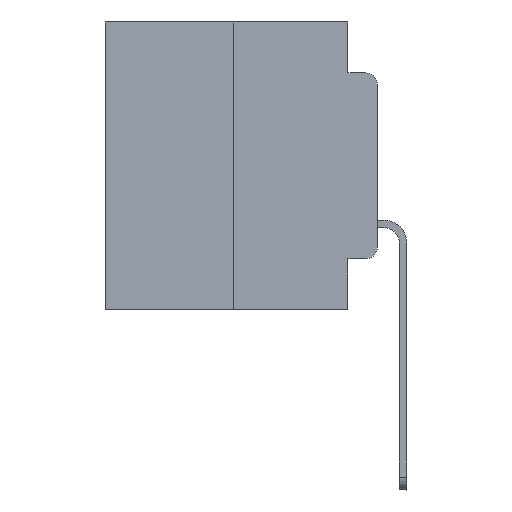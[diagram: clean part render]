
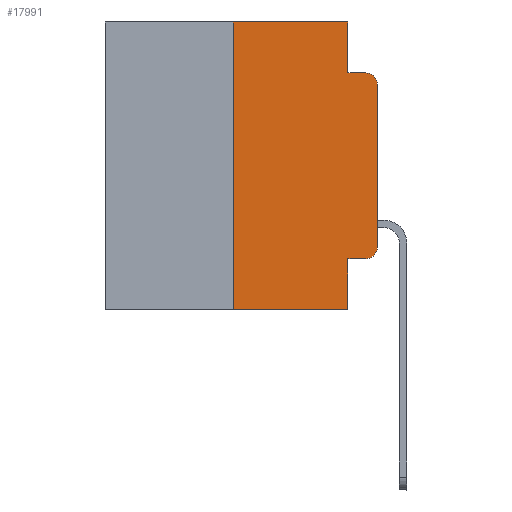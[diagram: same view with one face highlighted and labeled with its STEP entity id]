
A CAD part, left-side view. The second image highlights one B-rep face of the part: STEP entity #17991.
In plain terms, the highlighted planar face has unit normal (-1, 0, 0).
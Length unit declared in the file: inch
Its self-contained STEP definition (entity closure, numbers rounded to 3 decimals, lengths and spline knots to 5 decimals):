
#566 = CARTESIAN_POINT ( 'NONE',  ( 0., 0.051, 0. ) ) ;
#1534 = ORIENTED_EDGE ( 'NONE', *, *, #21400, .T. ) ;
#1569 = LINE ( 'NONE', #5666, #11738 ) ;
#3071 = CARTESIAN_POINT ( 'NONE',  ( 0., 0.02, -0.1085 ) ) ;
#3214 = DIRECTION ( 'NONE',  ( 0., -1., 0. ) ) ;
#3222 = DIRECTION ( 'NONE',  ( 0., 0., -1. ) ) ;
#3319 = VERTEX_POINT ( 'NONE', #20977 ) ;
#3355 = DIRECTION ( 'NONE',  ( -1., 0., 0. ) ) ;
#3459 = EDGE_CURVE ( 'NONE', #23044, #3319, #19981, .T. ) ;
#3983 = EDGE_CURVE ( 'NONE', #18690, #12984, #22580, .T. ) ;
#4078 = ORIENTED_EDGE ( 'NONE', *, *, #25641, .F. ) ;
#4236 = VECTOR ( 'NONE', #19928, 39.37008 ) ;
#4515 = DIRECTION ( 'NONE',  ( 0., 0., -1. ) ) ;
#4939 = CARTESIAN_POINT ( 'NONE',  ( 0., 0.25, 0. ) ) ;
#5666 = CARTESIAN_POINT ( 'NONE',  ( 0., 0.473, -0.5 ) ) ;
#6993 = ORIENTED_EDGE ( 'NONE', *, *, #23756, .F. ) ;
#7085 = CARTESIAN_POINT ( 'NONE',  ( 0., 0.051, -0.5 ) ) ;
#7463 = CARTESIAN_POINT ( 'NONE',  ( 0., 0., -0.3915 ) ) ;
#7580 = CARTESIAN_POINT ( 'NONE',  ( 0., 0.02, -0.4115 ) ) ;
#8139 = DIRECTION ( 'NONE',  ( 0., -1., 0. ) ) ;
#8253 = CARTESIAN_POINT ( 'NONE',  ( 0., 0.051, 0. ) ) ;
#8683 = EDGE_CURVE ( 'NONE', #12984, #23044, #17584, .T. ) ;
#8692 = FACE_OUTER_BOUND ( 'NONE', #15921, .T. ) ;
#8876 = CARTESIAN_POINT ( 'NONE',  ( 0., 0., 0. ) ) ;
#9052 = VECTOR ( 'NONE', #13506, 39.37008 ) ;
#9476 = ORIENTED_EDGE ( 'NONE', *, *, #20398, .F. ) ;
#9948 = CARTESIAN_POINT ( 'NONE',  ( 0., 0.051, -0.4115 ) ) ;
#10145 = DIRECTION ( 'NONE',  ( 0., -1., 0. ) ) ;
#10152 = VECTOR ( 'NONE', #3214, 39.37008 ) ;
#10549 = VECTOR ( 'NONE', #25100, 39.37008 ) ;
#10813 = DIRECTION ( 'NONE',  ( 1., 0., 0. ) ) ;
#10885 = VECTOR ( 'NONE', #4515, 39.37008 ) ;
#10991 = VECTOR ( 'NONE', #8139, 39.37008 ) ;
#11202 = LINE ( 'NONE', #20072, #4236 ) ;
#11250 = LINE ( 'NONE', #26156, #9052 ) ;
#11738 = VECTOR ( 'NONE', #10145, 39.37008 ) ;
#12093 = VERTEX_POINT ( 'NONE', #13845 ) ;
#12984 = VERTEX_POINT ( 'NONE', #7580 ) ;
#13320 = ORIENTED_EDGE ( 'NONE', *, *, #3983, .T. ) ;
#13492 = EDGE_CURVE ( 'NONE', #3319, #26957, #22589, .T. ) ;
#13506 = DIRECTION ( 'NONE',  ( 0., 0., 1. ) ) ;
#13530 = VERTEX_POINT ( 'NONE', #25093 ) ;
#13845 = CARTESIAN_POINT ( 'NONE',  ( 0., 0.051, -0.0885 ) ) ;
#14406 = EDGE_CURVE ( 'NONE', #12093, #26957, #22747, .T. ) ;
#15166 = DIRECTION ( 'NONE',  ( 0., 0., -1. ) ) ;
#15921 = EDGE_LOOP ( 'NONE', ( #25966, #27741, #21192, #4078, #9476, #27670, #1534, #6993, #13320, #22744 ) ) ;
#17306 = LINE ( 'NONE', #566, #10885 ) ;
#17584 = CIRCLE ( 'NONE', #18480, 0.02 ) ;
#17991 = ADVANCED_FACE ( 'NONE', ( #8692 ), #21895, .F. ) ;
#18480 = AXIS2_PLACEMENT_3D ( 'NONE', #24697, #3355, #3222 ) ;
#18690 = VERTEX_POINT ( 'NONE', #25208 ) ;
#19928 = DIRECTION ( 'NONE',  ( 0., -1., 0. ) ) ;
#19981 = LINE ( 'NONE', #8876, #20881 ) ;
#20072 = CARTESIAN_POINT ( 'NONE',  ( 0., 0.473, 0. ) ) ;
#20398 = EDGE_CURVE ( 'NONE', #21620, #13530, #11202, .T. ) ;
#20881 = VECTOR ( 'NONE', #24309, 39.37008 ) ;
#20908 = AXIS2_PLACEMENT_3D ( 'NONE', #27789, #10813, #15166 ) ;
#20977 = CARTESIAN_POINT ( 'NONE',  ( 0., 0., -0.1085 ) ) ;
#21192 = ORIENTED_EDGE ( 'NONE', *, *, #14406, .F. ) ;
#21400 = EDGE_CURVE ( 'NONE', #22997, #27542, #1569, .T. ) ;
#21620 = VERTEX_POINT ( 'NONE', #4939 ) ;
#21891 = DIRECTION ( 'NONE',  ( 0., 0., -1. ) ) ;
#21895 = PLANE ( 'NONE',  #20908 ) ;
#22580 = LINE ( 'NONE', #9948, #10152 ) ;
#22589 = CIRCLE ( 'NONE', #23028, 0.02 ) ;
#22744 = ORIENTED_EDGE ( 'NONE', *, *, #8683, .T. ) ;
#22747 = LINE ( 'NONE', #27389, #10991 ) ;
#22890 = EDGE_CURVE ( 'NONE', #22997, #21620, #11250, .T. ) ;
#22997 = VERTEX_POINT ( 'NONE', #24033 ) ;
#23028 = AXIS2_PLACEMENT_3D ( 'NONE', #3071, #26659, #21891 ) ;
#23044 = VERTEX_POINT ( 'NONE', #7463 ) ;
#23411 = LINE ( 'NONE', #8253, #10549 ) ;
#23756 = EDGE_CURVE ( 'NONE', #18690, #27542, #17306, .T. ) ;
#24033 = CARTESIAN_POINT ( 'NONE',  ( 0., 0.25, -0.5 ) ) ;
#24309 = DIRECTION ( 'NONE',  ( 0., 0., 1. ) ) ;
#24697 = CARTESIAN_POINT ( 'NONE',  ( 0., 0.02, -0.3915 ) ) ;
#25093 = CARTESIAN_POINT ( 'NONE',  ( 0., 0.051, 0. ) ) ;
#25100 = DIRECTION ( 'NONE',  ( 0., 0., -1. ) ) ;
#25208 = CARTESIAN_POINT ( 'NONE',  ( 0., 0.051, -0.4115 ) ) ;
#25393 = CARTESIAN_POINT ( 'NONE',  ( 0., 0.02, -0.0885 ) ) ;
#25641 = EDGE_CURVE ( 'NONE', #13530, #12093, #23411, .T. ) ;
#25966 = ORIENTED_EDGE ( 'NONE', *, *, #3459, .T. ) ;
#26156 = CARTESIAN_POINT ( 'NONE',  ( 0., 0.25, 0. ) ) ;
#26659 = DIRECTION ( 'NONE',  ( -1., 0., 0. ) ) ;
#26957 = VERTEX_POINT ( 'NONE', #25393 ) ;
#27389 = CARTESIAN_POINT ( 'NONE',  ( 0., 0.051, -0.0885 ) ) ;
#27542 = VERTEX_POINT ( 'NONE', #7085 ) ;
#27670 = ORIENTED_EDGE ( 'NONE', *, *, #22890, .F. ) ;
#27741 = ORIENTED_EDGE ( 'NONE', *, *, #13492, .T. ) ;
#27789 = CARTESIAN_POINT ( 'NONE',  ( 0., 0.473, 0. ) ) ;
